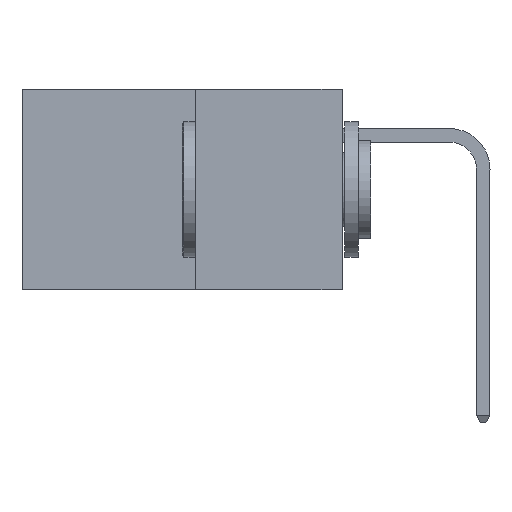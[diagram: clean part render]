
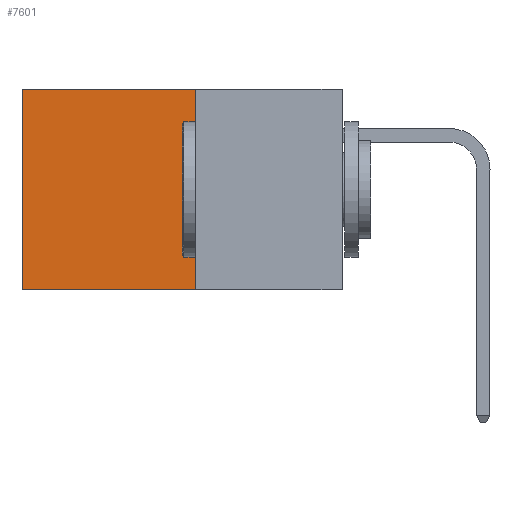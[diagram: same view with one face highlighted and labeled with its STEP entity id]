
A CAD part, left-side view. The second image highlights one B-rep face of the part: STEP entity #7601.
In plain terms, the highlighted planar face has unit normal (-1, 0, 0).
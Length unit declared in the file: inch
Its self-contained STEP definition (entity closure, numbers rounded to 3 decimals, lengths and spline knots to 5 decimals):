
#80 = CARTESIAN_POINT ( 'NONE',  ( 0.277, 0.59, -0.37 ) ) ;
#433 = EDGE_CURVE ( 'NONE', #1994, #26493, #10646, .T. ) ;
#1280 = ORIENTED_EDGE ( 'NONE', *, *, #24377, .F. ) ;
#1369 = DIRECTION ( 'NONE',  ( 0., 1., 0. ) ) ;
#1994 = VERTEX_POINT ( 'NONE', #20200 ) ;
#2564 = ORIENTED_EDGE ( 'NONE', *, *, #9918, .T. ) ;
#3111 = VERTEX_POINT ( 'NONE', #21231 ) ;
#3998 = CARTESIAN_POINT ( 'NONE',  ( 0.277, 0.27, -0.37 ) ) ;
#4488 = VERTEX_POINT ( 'NONE', #15687 ) ;
#5299 = LINE ( 'NONE', #20036, #26526 ) ;
#5541 = DIRECTION ( 'NONE',  ( 0., 0., -1. ) ) ;
#5851 = PLANE ( 'NONE',  #10461 ) ;
#7601 = ADVANCED_FACE ( 'NONE', ( #9068 ), #5851, .F. ) ;
#7943 = DIRECTION ( 'NONE',  ( 1., 0., 0. ) ) ;
#8549 = VECTOR ( 'NONE', #5541, 39.37008 ) ;
#9068 = FACE_OUTER_BOUND ( 'NONE', #16733, .T. ) ;
#9918 = EDGE_CURVE ( 'NONE', #4488, #26493, #10271, .T. ) ;
#9993 = VECTOR ( 'NONE', #16697, 39.37008 ) ;
#10271 = LINE ( 'NONE', #20699, #20658 ) ;
#10369 = DIRECTION ( 'NONE',  ( 0., 0., -1. ) ) ;
#10461 = AXIS2_PLACEMENT_3D ( 'NONE', #18294, #7943, #22447 ) ;
#10646 = LINE ( 'NONE', #3998, #9993 ) ;
#14310 = EDGE_CURVE ( 'NONE', #3111, #4488, #5299, .T. ) ;
#15687 = CARTESIAN_POINT ( 'NONE',  ( 0.277, 0.59, 0. ) ) ;
#16697 = DIRECTION ( 'NONE',  ( 0., 1., 0. ) ) ;
#16733 = EDGE_LOOP ( 'NONE', ( #2564, #18358, #1280, #19648 ) ) ;
#18294 = CARTESIAN_POINT ( 'NONE',  ( 0.277, 0.27, -0.37 ) ) ;
#18358 = ORIENTED_EDGE ( 'NONE', *, *, #433, .F. ) ;
#19596 = LINE ( 'NONE', #24059, #8549 ) ;
#19648 = ORIENTED_EDGE ( 'NONE', *, *, #14310, .T. ) ;
#20036 = CARTESIAN_POINT ( 'NONE',  ( 0.277, 0.27, 0. ) ) ;
#20200 = CARTESIAN_POINT ( 'NONE',  ( 0.277, 0.27, -0.37 ) ) ;
#20658 = VECTOR ( 'NONE', #10369, 39.37008 ) ;
#20699 = CARTESIAN_POINT ( 'NONE',  ( 0.277, 0.59, -0.37 ) ) ;
#21231 = CARTESIAN_POINT ( 'NONE',  ( 0.277, 0.27, 0. ) ) ;
#22447 = DIRECTION ( 'NONE',  ( 0., 0., -1. ) ) ;
#24059 = CARTESIAN_POINT ( 'NONE',  ( 0.277, 0.27, -0.37 ) ) ;
#24377 = EDGE_CURVE ( 'NONE', #3111, #1994, #19596, .T. ) ;
#26493 = VERTEX_POINT ( 'NONE', #80 ) ;
#26526 = VECTOR ( 'NONE', #1369, 39.37008 ) ;
